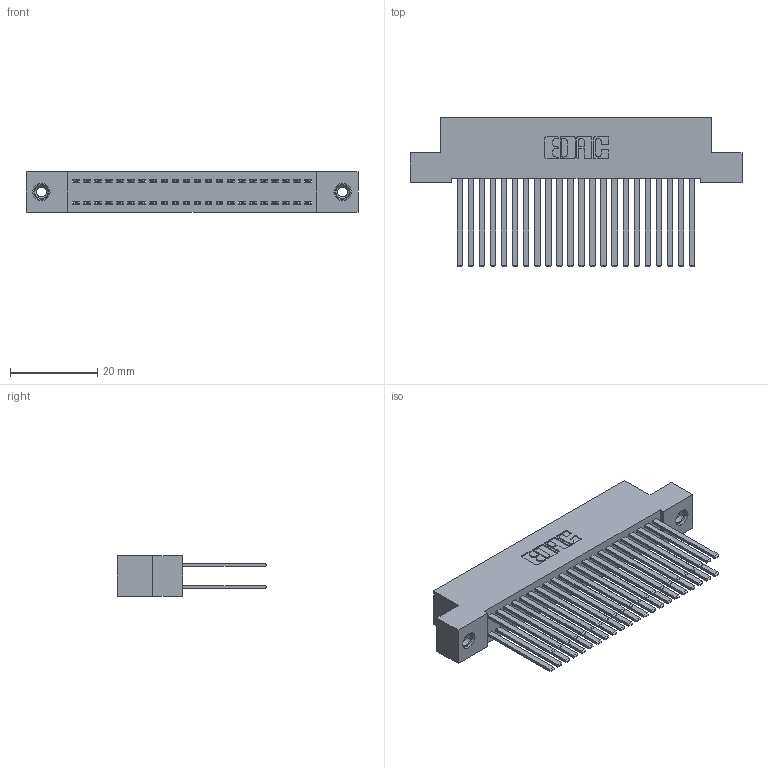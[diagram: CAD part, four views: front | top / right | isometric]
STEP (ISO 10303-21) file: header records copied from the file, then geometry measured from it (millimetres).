
FILE_DESCRIPTION (( 'STEP AP203' ), '1' );
FILE_NAME ('392-044-544-208.STEP', '2018-08-16T15:27:07', ( '' ), ( '' ), 'SwSTEP 2.0', 'SolidWorks 2016', '' );
FILE_SCHEMA (( 'CONFIG_CONTROL_DESIGN' ));
Length unit declared in the file: inch
Products named in the file (4): 342 Part_TI; 345-292-001_345-293-144; 345-250-001_345-250-003-102; 392-044-544-208
Assembly tree (47 placements, depth 2):
  392-044-544-208
    342 Part_TI
    345-292-001_345-293-144  x44
    345-250-001_345-250-003-102  x2
Bounding box: 76.2 x 34.3 x 9.4 mm (x, y, z)
Volume: 7363 mm3; surface area: 13210.7 mm2
Topology: 47 solids, 47 shells, 2194 faces, 6463 edges, 4242 vertices
Faces by surface type: plane 1506, cylinder 672, cone 12, torus 4
Entity records: 17610 total; most frequent: CARTESIAN_POINT 2921, ORIENTED_EDGE 2850, DIRECTION 2559, EDGE_CURVE 1425, VECTOR 1281, LINE 1281, VERTEX_POINT 944, AXIS2_PLACEMENT_3D 639
